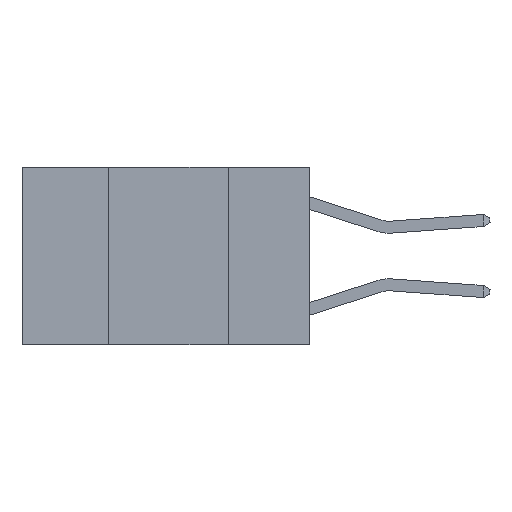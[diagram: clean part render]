
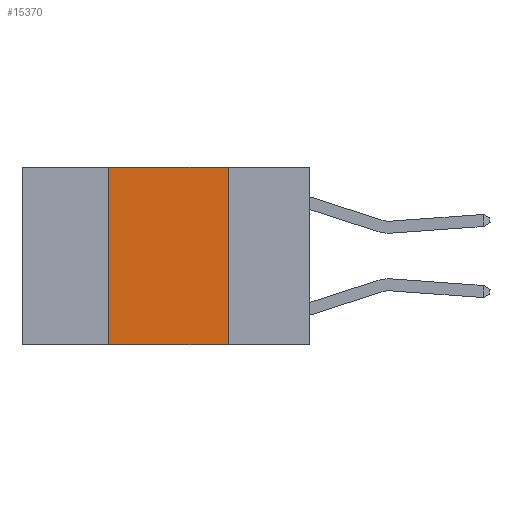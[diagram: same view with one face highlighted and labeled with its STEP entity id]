
A CAD part, left-side view. The second image highlights one B-rep face of the part: STEP entity #15370.
In plain terms, the highlighted planar face has unit normal (-1, 0, 0).
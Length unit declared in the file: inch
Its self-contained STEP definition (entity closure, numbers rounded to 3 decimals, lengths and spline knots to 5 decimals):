
#655 = DIRECTION ( 'NONE',  ( 0., 0., -1. ) ) ;
#804 = LINE ( 'NONE', #13662, #7667 ) ;
#1024 = CARTESIAN_POINT ( 'NONE',  ( 0., 0.42, -0.37 ) ) ;
#1037 = CARTESIAN_POINT ( 'NONE',  ( 0., 0.17, 0. ) ) ;
#1180 = EDGE_CURVE ( 'NONE', #11237, #5920, #11467, .T. ) ;
#1529 = ORIENTED_EDGE ( 'NONE', *, *, #4942, .T. ) ;
#1731 = LINE ( 'NONE', #5425, #2089 ) ;
#1853 = FACE_OUTER_BOUND ( 'NONE', #3168, .T. ) ;
#2089 = VECTOR ( 'NONE', #2921, 39.37008 ) ;
#2568 = DIRECTION ( 'NONE',  ( 0., 0., -1. ) ) ;
#2921 = DIRECTION ( 'NONE',  ( 0., -1., 0. ) ) ;
#3168 = EDGE_LOOP ( 'NONE', ( #4181, #12164, #9664, #1529 ) ) ;
#4181 = ORIENTED_EDGE ( 'NONE', *, *, #16484, .F. ) ;
#4335 = CARTESIAN_POINT ( 'NONE',  ( 0., 0.6, 0. ) ) ;
#4700 = VECTOR ( 'NONE', #2568, 39.37008 ) ;
#4942 = EDGE_CURVE ( 'NONE', #11237, #16838, #1731, .T. ) ;
#5425 = CARTESIAN_POINT ( 'NONE',  ( 0., 0.6, -0.37 ) ) ;
#5776 = AXIS2_PLACEMENT_3D ( 'NONE', #4335, #12403, #655 ) ;
#5920 = VERTEX_POINT ( 'NONE', #12796 ) ;
#6259 = LINE ( 'NONE', #1037, #4700 ) ;
#6725 = CARTESIAN_POINT ( 'NONE',  ( 0., 0.42, 0. ) ) ;
#7151 = DIRECTION ( 'NONE',  ( 0., -1., 0. ) ) ;
#7600 = DIRECTION ( 'NONE',  ( 0., 0., 1. ) ) ;
#7667 = VECTOR ( 'NONE', #7151, 39.37008 ) ;
#8206 = PLANE ( 'NONE',  #5776 ) ;
#8424 = EDGE_CURVE ( 'NONE', #5920, #16274, #804, .T. ) ;
#9664 = ORIENTED_EDGE ( 'NONE', *, *, #1180, .F. ) ;
#11237 = VERTEX_POINT ( 'NONE', #1024 ) ;
#11467 = LINE ( 'NONE', #6725, #15872 ) ;
#12020 = CARTESIAN_POINT ( 'NONE',  ( 0., 0.17, 0. ) ) ;
#12164 = ORIENTED_EDGE ( 'NONE', *, *, #8424, .F. ) ;
#12403 = DIRECTION ( 'NONE',  ( 1., 0., 0. ) ) ;
#12796 = CARTESIAN_POINT ( 'NONE',  ( 0., 0.42, 0. ) ) ;
#13662 = CARTESIAN_POINT ( 'NONE',  ( 0., 0.6, 0. ) ) ;
#15370 = ADVANCED_FACE ( 'NONE', ( #1853 ), #8206, .F. ) ;
#15399 = CARTESIAN_POINT ( 'NONE',  ( 0., 0.17, -0.37 ) ) ;
#15872 = VECTOR ( 'NONE', #7600, 39.37008 ) ;
#16274 = VERTEX_POINT ( 'NONE', #12020 ) ;
#16484 = EDGE_CURVE ( 'NONE', #16274, #16838, #6259, .T. ) ;
#16838 = VERTEX_POINT ( 'NONE', #15399 ) ;
